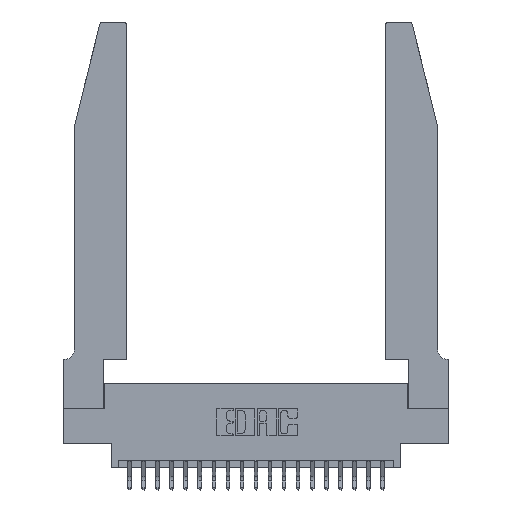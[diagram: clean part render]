
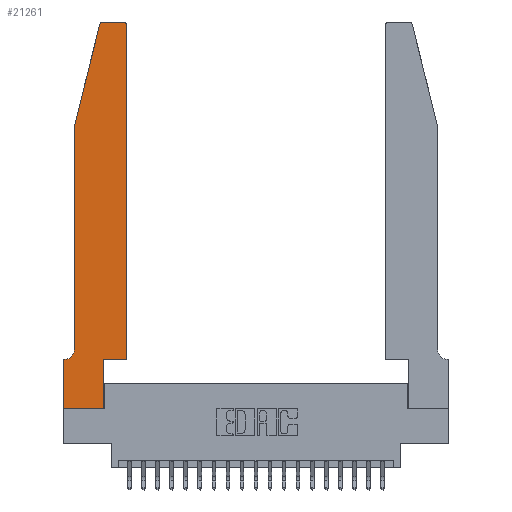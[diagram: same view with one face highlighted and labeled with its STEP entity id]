
A CAD part, top view. The second image highlights one B-rep face of the part: STEP entity #21261.
In plain terms, the highlighted planar face has unit normal (0, 0, 1).
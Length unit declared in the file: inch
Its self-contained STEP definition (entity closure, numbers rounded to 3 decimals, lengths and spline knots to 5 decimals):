
#655 = DIRECTION ( 'NONE',  ( 0., -1., 0. ) ) ;
#805 = CIRCLE ( 'NONE', #8937, 0.07 ) ;
#1021 = DIRECTION ( 'NONE',  ( -0.239, -0.971, 0. ) ) ;
#1066 = DIRECTION ( 'NONE',  ( 0., -1., 0. ) ) ;
#1700 = LINE ( 'NONE', #22404, #15602 ) ;
#1815 = DIRECTION ( 'NONE',  ( 1., 0., 0. ) ) ;
#2385 = VECTOR ( 'NONE', #10683, 39.37008 ) ;
#2672 = ORIENTED_EDGE ( 'NONE', *, *, #11992, .T. ) ;
#2676 = VERTEX_POINT ( 'NONE', #11923 ) ;
#2685 = CARTESIAN_POINT ( 'NONE',  ( 0.4505, 2.72, 0.37 ) ) ;
#2784 = EDGE_CURVE ( 'NONE', #17601, #12048, #15540, .T. ) ;
#3564 = EDGE_CURVE ( 'NONE', #12163, #5470, #14698, .T. ) ;
#3743 = VECTOR ( 'NONE', #655, 39.37008 ) ;
#4313 = DIRECTION ( 'NONE',  ( 0., 0., 1. ) ) ;
#4444 = ORIENTED_EDGE ( 'NONE', *, *, #11257, .T. ) ;
#5000 = CARTESIAN_POINT ( 'NONE',  ( 0.4505, 0.35, 0.37 ) ) ;
#5094 = CARTESIAN_POINT ( 'NONE',  ( 0.0055, 0.35, 0.37 ) ) ;
#5140 = VECTOR ( 'NONE', #20776, 39.37008 ) ;
#5255 = CARTESIAN_POINT ( 'NONE',  ( 0.2865, 0., 0.37 ) ) ;
#5437 = DIRECTION ( 'NONE',  ( 0., 0., -1. ) ) ;
#5470 = VERTEX_POINT ( 'NONE', #20520 ) ;
#5486 = CARTESIAN_POINT ( 'NONE',  ( 0., 0.35, 0.37 ) ) ;
#5739 = CIRCLE ( 'NONE', #12749, 0.03 ) ;
#5812 = ORIENTED_EDGE ( 'NONE', *, *, #2784, .T. ) ;
#5969 = CARTESIAN_POINT ( 'NONE',  ( 0.0755, 2., 0.37 ) ) ;
#6030 = LINE ( 'NONE', #7820, #15572 ) ;
#6410 = ORIENTED_EDGE ( 'NONE', *, *, #21014, .T. ) ;
#6798 = LINE ( 'NONE', #5000, #20911 ) ;
#6832 = ORIENTED_EDGE ( 'NONE', *, *, #11818, .T. ) ;
#6978 = AXIS2_PLACEMENT_3D ( 'NONE', #15095, #4313, #16870 ) ;
#7293 = LINE ( 'NONE', #17702, #2385 ) ;
#7626 = EDGE_LOOP ( 'NONE', ( #21232, #6832, #6410, #5812, #19673, #19819, #4444, #2672, #10018, #19370, #18228, #11088 ) ) ;
#7820 = CARTESIAN_POINT ( 'NONE',  ( 0.0755, 0.35, 0.37 ) ) ;
#8031 = LINE ( 'NONE', #22068, #3743 ) ;
#8469 = CARTESIAN_POINT ( 'NONE',  ( 0., 0., 0.37 ) ) ;
#8696 = EDGE_CURVE ( 'NONE', #5470, #11919, #7293, .T. ) ;
#8851 = LINE ( 'NONE', #8469, #5140 ) ;
#8937 = AXIS2_PLACEMENT_3D ( 'NONE', #16175, #5437, #17948 ) ;
#9120 = LINE ( 'NONE', #19648, #13336 ) ;
#9617 = VERTEX_POINT ( 'NONE', #22054 ) ;
#10018 = ORIENTED_EDGE ( 'NONE', *, *, #3564, .T. ) ;
#10034 = FACE_OUTER_BOUND ( 'NONE', #7626, .T. ) ;
#10248 = CARTESIAN_POINT ( 'NONE',  ( 0.4205, 2.72, 0.37 ) ) ;
#10341 = CARTESIAN_POINT ( 'NONE',  ( 0.0755, 2., 0.37 ) ) ;
#10683 = DIRECTION ( 'NONE',  ( 1., 0., 0. ) ) ;
#10901 = CARTESIAN_POINT ( 'NONE',  ( 0.25487, 2.72718, 0.37 ) ) ;
#10923 = DIRECTION ( 'NONE',  ( -1., 0., 0. ) ) ;
#10941 = VERTEX_POINT ( 'NONE', #10901 ) ;
#11088 = ORIENTED_EDGE ( 'NONE', *, *, #11398, .T. ) ;
#11257 = EDGE_CURVE ( 'NONE', #13204, #9617, #8031, .T. ) ;
#11398 = EDGE_CURVE ( 'NONE', #16659, #2676, #5739, .T. ) ;
#11818 = EDGE_CURVE ( 'NONE', #21038, #10941, #20967, .T. ) ;
#11919 = VERTEX_POINT ( 'NONE', #17013 ) ;
#11923 = CARTESIAN_POINT ( 'NONE',  ( 0.4205, 2.75, 0.37 ) ) ;
#11992 = EDGE_CURVE ( 'NONE', #9617, #12163, #8851, .T. ) ;
#12048 = VERTEX_POINT ( 'NONE', #22628 ) ;
#12054 = DIRECTION ( 'NONE',  ( 1., 0., 0. ) ) ;
#12163 = VERTEX_POINT ( 'NONE', #5255 ) ;
#12246 = EDGE_CURVE ( 'NONE', #2676, #21038, #9120, .T. ) ;
#12749 = AXIS2_PLACEMENT_3D ( 'NONE', #10248, #22438, #12054 ) ;
#12785 = DIRECTION ( 'NONE',  ( 0., 0., 1. ) ) ;
#13204 = VERTEX_POINT ( 'NONE', #19385 ) ;
#13308 = EDGE_CURVE ( 'NONE', #11919, #16659, #6798, .T. ) ;
#13336 = VECTOR ( 'NONE', #10923, 39.37008 ) ;
#14477 = PLANE ( 'NONE',  #17593 ) ;
#14506 = DIRECTION ( 'NONE',  ( 0., 1., 0. ) ) ;
#14698 = LINE ( 'NONE', #21379, #18792 ) ;
#15095 = CARTESIAN_POINT ( 'NONE',  ( 0.284, 2.72, 0.37 ) ) ;
#15540 = LINE ( 'NONE', #10341, #19095 ) ;
#15572 = VECTOR ( 'NONE', #20182, 39.37008 ) ;
#15602 = VECTOR ( 'NONE', #1021, 39.37008 ) ;
#16175 = CARTESIAN_POINT ( 'NONE',  ( 0.0055, 0.42, 0.37 ) ) ;
#16659 = VERTEX_POINT ( 'NONE', #2685 ) ;
#16870 = DIRECTION ( 'NONE',  ( 1., 0., 0. ) ) ;
#17013 = CARTESIAN_POINT ( 'NONE',  ( 0.4505, 0.35, 0.37 ) ) ;
#17593 = AXIS2_PLACEMENT_3D ( 'NONE', #5486, #12785, #1815 ) ;
#17601 = VERTEX_POINT ( 'NONE', #5969 ) ;
#17702 = CARTESIAN_POINT ( 'NONE',  ( 0.4505, 0.35, 0.37 ) ) ;
#17948 = DIRECTION ( 'NONE',  ( -1., 0., 0. ) ) ;
#18228 = ORIENTED_EDGE ( 'NONE', *, *, #13308, .T. ) ;
#18792 = VECTOR ( 'NONE', #14506, 39.37008 ) ;
#19095 = VECTOR ( 'NONE', #1066, 39.37008 ) ;
#19172 = VERTEX_POINT ( 'NONE', #5094 ) ;
#19370 = ORIENTED_EDGE ( 'NONE', *, *, #8696, .T. ) ;
#19385 = CARTESIAN_POINT ( 'NONE',  ( 0., 0.35, 0.37 ) ) ;
#19648 = CARTESIAN_POINT ( 'NONE',  ( 0.2605, 2.75, 0.37 ) ) ;
#19673 = ORIENTED_EDGE ( 'NONE', *, *, #20583, .T. ) ;
#19819 = ORIENTED_EDGE ( 'NONE', *, *, #20798, .T. ) ;
#20182 = DIRECTION ( 'NONE',  ( -1., 0., 0. ) ) ;
#20520 = CARTESIAN_POINT ( 'NONE',  ( 0.2865, 0.35, 0.37 ) ) ;
#20583 = EDGE_CURVE ( 'NONE', #12048, #19172, #805, .T. ) ;
#20776 = DIRECTION ( 'NONE',  ( 1., 0., 0. ) ) ;
#20798 = EDGE_CURVE ( 'NONE', #19172, #13204, #6030, .T. ) ;
#20911 = VECTOR ( 'NONE', #22916, 39.37008 ) ;
#20967 = CIRCLE ( 'NONE', #6978, 0.03 ) ;
#21014 = EDGE_CURVE ( 'NONE', #10941, #17601, #1700, .T. ) ;
#21038 = VERTEX_POINT ( 'NONE', #22485 ) ;
#21232 = ORIENTED_EDGE ( 'NONE', *, *, #12246, .T. ) ;
#21261 = ADVANCED_FACE ( 'NONE', ( #10034 ), #14477, .T. ) ;
#21379 = CARTESIAN_POINT ( 'NONE',  ( 0.2865, 0.35, 0.37 ) ) ;
#22054 = CARTESIAN_POINT ( 'NONE',  ( 0., 0., 0.37 ) ) ;
#22068 = CARTESIAN_POINT ( 'NONE',  ( 0., 0., 0.37 ) ) ;
#22404 = CARTESIAN_POINT ( 'NONE',  ( 0.0755, 2., 0.37 ) ) ;
#22438 = DIRECTION ( 'NONE',  ( 0., 0., 1. ) ) ;
#22485 = CARTESIAN_POINT ( 'NONE',  ( 0.284, 2.75, 0.37 ) ) ;
#22628 = CARTESIAN_POINT ( 'NONE',  ( 0.0755, 0.42, 0.37 ) ) ;
#22916 = DIRECTION ( 'NONE',  ( 0., 1., 0. ) ) ;
